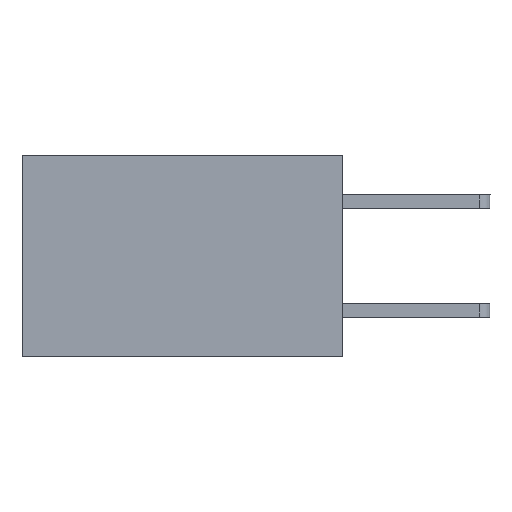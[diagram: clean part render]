
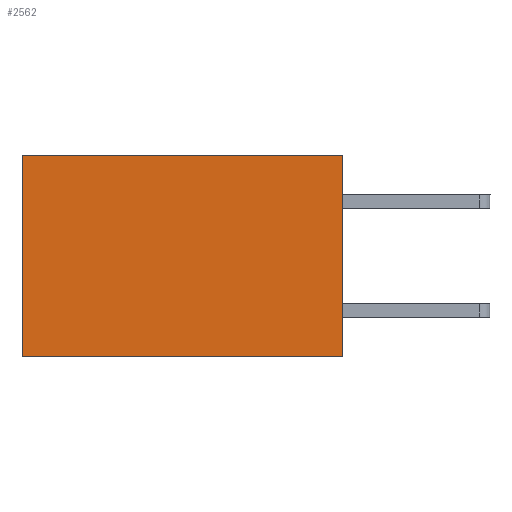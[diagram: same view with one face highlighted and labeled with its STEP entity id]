
A CAD part, left-side view. The second image highlights one B-rep face of the part: STEP entity #2562.
In plain terms, the highlighted planar face has unit normal (-1, 0, 0).
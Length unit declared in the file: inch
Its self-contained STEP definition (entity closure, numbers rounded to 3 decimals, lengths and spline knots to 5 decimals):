
#350 = ORIENTED_EDGE ( 'NONE', *, *, #4553, .F. ) ;
#422 = EDGE_CURVE ( 'NONE', #3052, #662, #3471, .T. ) ;
#662 = VERTEX_POINT ( 'NONE', #2242 ) ;
#781 = AXIS2_PLACEMENT_3D ( 'NONE', #2579, #2500, #1439 ) ;
#889 = CARTESIAN_POINT ( 'NONE',  ( 0.277, 0., -0.37 ) ) ;
#895 = VERTEX_POINT ( 'NONE', #3115 ) ;
#1000 = CARTESIAN_POINT ( 'NONE',  ( 0.277, 0., -0.37 ) ) ;
#1258 = EDGE_CURVE ( 'NONE', #895, #3052, #2499, .T. ) ;
#1413 = ORIENTED_EDGE ( 'NONE', *, *, #1258, .T. ) ;
#1439 = DIRECTION ( 'NONE',  ( 0., 0., -1. ) ) ;
#1702 = LINE ( 'NONE', #889, #1922 ) ;
#1922 = VECTOR ( 'NONE', #3201, 39.37008 ) ;
#2015 = CARTESIAN_POINT ( 'NONE',  ( 0.277, 0., 0. ) ) ;
#2097 = LINE ( 'NONE', #1000, #2955 ) ;
#2242 = CARTESIAN_POINT ( 'NONE',  ( 0.277, 0.59, -0.37 ) ) ;
#2492 = ORIENTED_EDGE ( 'NONE', *, *, #422, .T. ) ;
#2499 = LINE ( 'NONE', #2015, #6191 ) ;
#2500 = DIRECTION ( 'NONE',  ( 1., 0., 0. ) ) ;
#2562 = ADVANCED_FACE ( 'NONE', ( #6617 ), #4860, .F. ) ;
#2579 = CARTESIAN_POINT ( 'NONE',  ( 0.277, 0., -0.37 ) ) ;
#2955 = VECTOR ( 'NONE', #3919, 39.37008 ) ;
#3028 = VECTOR ( 'NONE', #4484, 39.37008 ) ;
#3052 = VERTEX_POINT ( 'NONE', #5529 ) ;
#3115 = CARTESIAN_POINT ( 'NONE',  ( 0.277, 0., 0. ) ) ;
#3201 = DIRECTION ( 'NONE',  ( 0., 1., 0. ) ) ;
#3263 = CARTESIAN_POINT ( 'NONE',  ( 0.277, 0., -0.37 ) ) ;
#3471 = LINE ( 'NONE', #6375, #3028 ) ;
#3655 = VERTEX_POINT ( 'NONE', #3263 ) ;
#3683 = DIRECTION ( 'NONE',  ( 0., 1., 0. ) ) ;
#3919 = DIRECTION ( 'NONE',  ( 0., 0., -1. ) ) ;
#4484 = DIRECTION ( 'NONE',  ( 0., 0., -1. ) ) ;
#4553 = EDGE_CURVE ( 'NONE', #3655, #662, #1702, .T. ) ;
#4860 = PLANE ( 'NONE',  #781 ) ;
#5529 = CARTESIAN_POINT ( 'NONE',  ( 0.277, 0.59, 0. ) ) ;
#5782 = EDGE_LOOP ( 'NONE', ( #2492, #350, #6763, #1413 ) ) ;
#6191 = VECTOR ( 'NONE', #3683, 39.37008 ) ;
#6316 = EDGE_CURVE ( 'NONE', #895, #3655, #2097, .T. ) ;
#6375 = CARTESIAN_POINT ( 'NONE',  ( 0.277, 0.59, -0.37 ) ) ;
#6617 = FACE_OUTER_BOUND ( 'NONE', #5782, .T. ) ;
#6763 = ORIENTED_EDGE ( 'NONE', *, *, #6316, .F. ) ;
